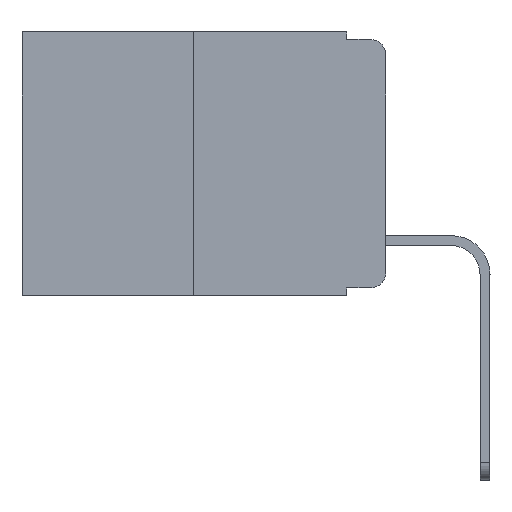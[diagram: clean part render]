
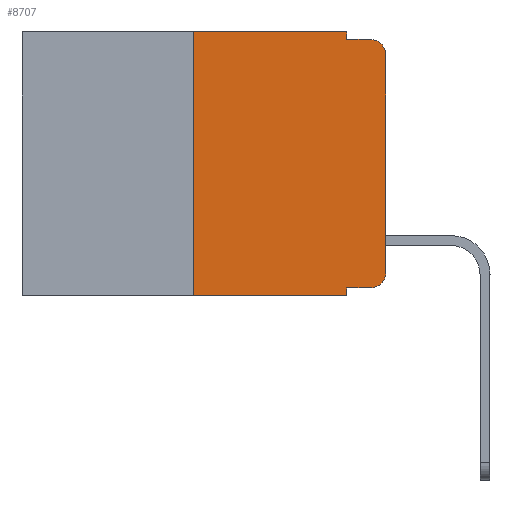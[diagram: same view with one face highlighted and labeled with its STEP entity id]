
A CAD part, left-side view. The second image highlights one B-rep face of the part: STEP entity #8707.
In plain terms, the highlighted planar face has unit normal (-1, 0, 0).
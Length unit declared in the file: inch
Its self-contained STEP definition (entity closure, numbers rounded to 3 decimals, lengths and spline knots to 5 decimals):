
#71 = VERTEX_POINT ( 'NONE', #352 ) ;
#78 = LINE ( 'NONE', #640, #6571 ) ;
#352 = CARTESIAN_POINT ( 'NONE',  ( 0., 0.051, 0. ) ) ;
#427 = VECTOR ( 'NONE', #6479, 39.37008 ) ;
#439 = CARTESIAN_POINT ( 'NONE',  ( 0., 0.051, 0. ) ) ;
#640 = CARTESIAN_POINT ( 'NONE',  ( 0., 0.051, -0.01 ) ) ;
#778 = LINE ( 'NONE', #13177, #2610 ) ;
#1144 = EDGE_CURVE ( 'NONE', #71, #4748, #13597, .T. ) ;
#1383 = DIRECTION ( 'NONE',  ( -1., 0., 0. ) ) ;
#1463 = VERTEX_POINT ( 'NONE', #4655 ) ;
#1575 = ORIENTED_EDGE ( 'NONE', *, *, #3120, .F. ) ;
#1695 = VECTOR ( 'NONE', #10778, 39.37008 ) ;
#2101 = ORIENTED_EDGE ( 'NONE', *, *, #3413, .T. ) ;
#2357 = CARTESIAN_POINT ( 'NONE',  ( 0., 0.02, -0.03 ) ) ;
#2511 = EDGE_CURVE ( 'NONE', #11011, #13062, #13736, .T. ) ;
#2610 = VECTOR ( 'NONE', #7889, 39.37008 ) ;
#2620 = EDGE_CURVE ( 'NONE', #1463, #3090, #778, .T. ) ;
#2631 = AXIS2_PLACEMENT_3D ( 'NONE', #7482, #8521, #5241 ) ;
#2642 = CARTESIAN_POINT ( 'NONE',  ( 0., 0.473, -0.343 ) ) ;
#2673 = EDGE_CURVE ( 'NONE', #6569, #11011, #11739, .T. ) ;
#2846 = EDGE_LOOP ( 'NONE', ( #3486, #9409, #5469, #10233, #1575, #11920, #2101, #12879, #8485, #12063 ) ) ;
#3090 = VERTEX_POINT ( 'NONE', #5668 ) ;
#3103 = VECTOR ( 'NONE', #4899, 39.37008 ) ;
#3120 = EDGE_CURVE ( 'NONE', #3090, #71, #13212, .T. ) ;
#3173 = LINE ( 'NONE', #11816, #1695 ) ;
#3413 = EDGE_CURVE ( 'NONE', #1463, #13701, #3764, .T. ) ;
#3486 = ORIENTED_EDGE ( 'NONE', *, *, #2673, .T. ) ;
#3511 = EDGE_CURVE ( 'NONE', #4748, #13062, #78, .T. ) ;
#3764 = LINE ( 'NONE', #2642, #3103 ) ;
#4309 = CIRCLE ( 'NONE', #7424, 0.02 ) ;
#4655 = CARTESIAN_POINT ( 'NONE',  ( 0., 0.25, -0.343 ) ) ;
#4748 = VERTEX_POINT ( 'NONE', #10679 ) ;
#4899 = DIRECTION ( 'NONE',  ( 0., -1., 0. ) ) ;
#4936 = VECTOR ( 'NONE', #12183, 39.37008 ) ;
#5018 = CARTESIAN_POINT ( 'NONE',  ( 0., 0.02, -0.01 ) ) ;
#5083 = CARTESIAN_POINT ( 'NONE',  ( 0., 0.051, -0.343 ) ) ;
#5188 = CARTESIAN_POINT ( 'NONE',  ( 0., 0.051, 0. ) ) ;
#5241 = DIRECTION ( 'NONE',  ( 0., 0., -1. ) ) ;
#5314 = CARTESIAN_POINT ( 'NONE',  ( 0., 0.473, 0. ) ) ;
#5449 = VERTEX_POINT ( 'NONE', #12312 ) ;
#5469 = ORIENTED_EDGE ( 'NONE', *, *, #3511, .F. ) ;
#5668 = CARTESIAN_POINT ( 'NONE',  ( 0., 0.25, 0. ) ) ;
#5999 = CARTESIAN_POINT ( 'NONE',  ( 0., 0.02, -0.313 ) ) ;
#6338 = EDGE_CURVE ( 'NONE', #5449, #11423, #3173, .T. ) ;
#6479 = DIRECTION ( 'NONE',  ( 0., -1., 0. ) ) ;
#6569 = VERTEX_POINT ( 'NONE', #10117 ) ;
#6571 = VECTOR ( 'NONE', #13447, 39.37008 ) ;
#7284 = VECTOR ( 'NONE', #11503, 39.37008 ) ;
#7424 = AXIS2_PLACEMENT_3D ( 'NONE', #5999, #13397, #9178 ) ;
#7482 = CARTESIAN_POINT ( 'NONE',  ( 0., 0.473, 0. ) ) ;
#7889 = DIRECTION ( 'NONE',  ( 0., 0., 1. ) ) ;
#8135 = AXIS2_PLACEMENT_3D ( 'NONE', #2357, #1383, #9806 ) ;
#8485 = ORIENTED_EDGE ( 'NONE', *, *, #6338, .T. ) ;
#8521 = DIRECTION ( 'NONE',  ( 1., 0., 0. ) ) ;
#8707 = ADVANCED_FACE ( 'NONE', ( #11468 ), #11703, .F. ) ;
#9068 = DIRECTION ( 'NONE',  ( 0., 0., -1. ) ) ;
#9097 = EDGE_CURVE ( 'NONE', #11423, #6569, #4309, .T. ) ;
#9178 = DIRECTION ( 'NONE',  ( 0., 0., -1. ) ) ;
#9409 = ORIENTED_EDGE ( 'NONE', *, *, #2511, .T. ) ;
#9588 = CARTESIAN_POINT ( 'NONE',  ( 0., 0., -0.03 ) ) ;
#9806 = DIRECTION ( 'NONE',  ( 0., 0., -1. ) ) ;
#10117 = CARTESIAN_POINT ( 'NONE',  ( 0., 0., -0.313 ) ) ;
#10233 = ORIENTED_EDGE ( 'NONE', *, *, #1144, .F. ) ;
#10679 = CARTESIAN_POINT ( 'NONE',  ( 0., 0.051, -0.01 ) ) ;
#10778 = DIRECTION ( 'NONE',  ( 0., -1., 0. ) ) ;
#10999 = CARTESIAN_POINT ( 'NONE',  ( 0., 0., 0. ) ) ;
#11011 = VERTEX_POINT ( 'NONE', #9588 ) ;
#11423 = VERTEX_POINT ( 'NONE', #11547 ) ;
#11468 = FACE_OUTER_BOUND ( 'NONE', #2846, .T. ) ;
#11503 = DIRECTION ( 'NONE',  ( 0., 0., -1. ) ) ;
#11547 = CARTESIAN_POINT ( 'NONE',  ( 0., 0.02, -0.333 ) ) ;
#11703 = PLANE ( 'NONE',  #2631 ) ;
#11739 = LINE ( 'NONE', #10999, #4936 ) ;
#11816 = CARTESIAN_POINT ( 'NONE',  ( 0., 0.051, -0.333 ) ) ;
#11920 = ORIENTED_EDGE ( 'NONE', *, *, #2620, .F. ) ;
#12063 = ORIENTED_EDGE ( 'NONE', *, *, #9097, .T. ) ;
#12183 = DIRECTION ( 'NONE',  ( 0., 0., 1. ) ) ;
#12312 = CARTESIAN_POINT ( 'NONE',  ( 0., 0.051, -0.333 ) ) ;
#12879 = ORIENTED_EDGE ( 'NONE', *, *, #13526, .F. ) ;
#13062 = VERTEX_POINT ( 'NONE', #5018 ) ;
#13177 = CARTESIAN_POINT ( 'NONE',  ( 0., 0.25, 0. ) ) ;
#13212 = LINE ( 'NONE', #5314, #427 ) ;
#13390 = VECTOR ( 'NONE', #9068, 39.37008 ) ;
#13397 = DIRECTION ( 'NONE',  ( -1., 0., 0. ) ) ;
#13447 = DIRECTION ( 'NONE',  ( 0., -1., 0. ) ) ;
#13526 = EDGE_CURVE ( 'NONE', #5449, #13701, #13740, .T. ) ;
#13597 = LINE ( 'NONE', #5188, #7284 ) ;
#13701 = VERTEX_POINT ( 'NONE', #5083 ) ;
#13736 = CIRCLE ( 'NONE', #8135, 0.02 ) ;
#13740 = LINE ( 'NONE', #439, #13390 ) ;
